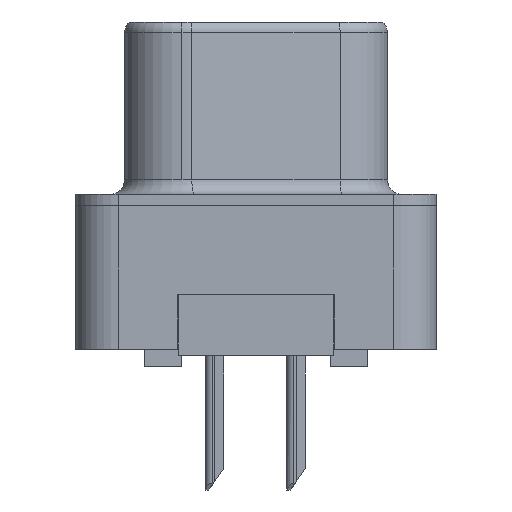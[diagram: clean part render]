
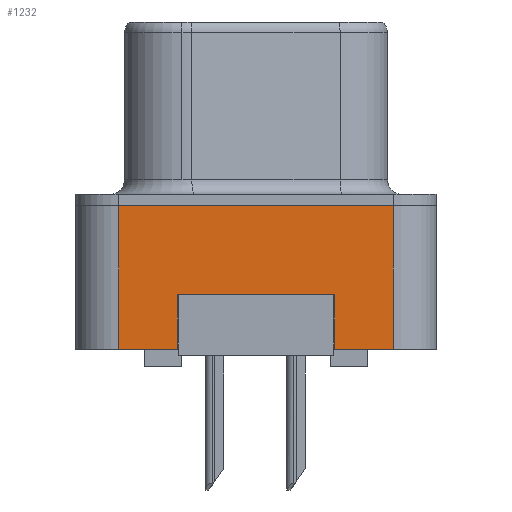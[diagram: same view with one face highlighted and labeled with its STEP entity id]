
A CAD part, left-side view. The second image highlights one B-rep face of the part: STEP entity #1232.
In plain terms, the highlighted planar face has unit normal (-1, 0, 0).
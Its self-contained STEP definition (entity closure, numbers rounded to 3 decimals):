
#212 = CARTESIAN_POINT ( 'NONE',  ( -3., -2.75, -3.1 ) ) ;
#1232 = ADVANCED_FACE ( 'NONE', ( #14462 ), #5292, .T. ) ;
#1903 = DIRECTION ( 'NONE',  ( 0., 0., -1. ) ) ;
#2161 = EDGE_CURVE ( 'NONE', #9326, #15924, #23669, .T. ) ;
#2201 = EDGE_CURVE ( 'NONE', #21811, #5890, #8707, .T. ) ;
#2222 = ORIENTED_EDGE ( 'NONE', *, *, #4855, .F. ) ;
#2808 = ORIENTED_EDGE ( 'NONE', *, *, #2161, .T. ) ;
#3086 = CARTESIAN_POINT ( 'NONE',  ( -3., -4.775, -5. ) ) ;
#3478 = VERTEX_POINT ( 'NONE', #15378 ) ;
#3580 = CARTESIAN_POINT ( 'NONE',  ( -3., 4.775, -5. ) ) ;
#3898 = ORIENTED_EDGE ( 'NONE', *, *, #20613, .T. ) ;
#4206 = DIRECTION ( 'NONE',  ( 0., -1., 0. ) ) ;
#4207 = CARTESIAN_POINT ( 'NONE',  ( -3., 4.775, -5. ) ) ;
#4543 = DIRECTION ( 'NONE',  ( 0., -1., 0. ) ) ;
#4855 = EDGE_CURVE ( 'NONE', #9326, #3478, #13687, .T. ) ;
#5292 = PLANE ( 'NONE',  #23147 ) ;
#5328 = ORIENTED_EDGE ( 'NONE', *, *, #14729, .F. ) ;
#5890 = VERTEX_POINT ( 'NONE', #11511 ) ;
#6472 = VERTEX_POINT ( 'NONE', #3580 ) ;
#7315 = VECTOR ( 'NONE', #11886, 1000. ) ;
#8707 = LINE ( 'NONE', #16070, #13451 ) ;
#8901 = CARTESIAN_POINT ( 'NONE',  ( -3., -4.775, -5. ) ) ;
#9162 = LINE ( 'NONE', #14600, #19308 ) ;
#9326 = VERTEX_POINT ( 'NONE', #212 ) ;
#9876 = LINE ( 'NONE', #15428, #13224 ) ;
#9992 = LINE ( 'NONE', #4207, #16494 ) ;
#11348 = EDGE_LOOP ( 'NONE', ( #2808, #12873, #16657, #22476, #5328, #3898, #13068, #2222 ) ) ;
#11511 = CARTESIAN_POINT ( 'NONE',  ( -3., -4.775, 0. ) ) ;
#11766 = CARTESIAN_POINT ( 'NONE',  ( -3., 2.75, -3.1 ) ) ;
#11886 = DIRECTION ( 'NONE',  ( 0., 1., 0. ) ) ;
#12662 = DIRECTION ( 'NONE',  ( 0., -1., 0. ) ) ;
#12873 = ORIENTED_EDGE ( 'NONE', *, *, #17769, .T. ) ;
#13068 = ORIENTED_EDGE ( 'NONE', *, *, #22928, .F. ) ;
#13224 = VECTOR ( 'NONE', #4206, 1000. ) ;
#13404 = CARTESIAN_POINT ( 'NONE',  ( -3., 4.775, 0. ) ) ;
#13451 = VECTOR ( 'NONE', #23436, 1000. ) ;
#13486 = CARTESIAN_POINT ( 'NONE',  ( -3., -2.75, -5. ) ) ;
#13687 = LINE ( 'NONE', #11766, #7315 ) ;
#14462 = FACE_OUTER_BOUND ( 'NONE', #11348, .T. ) ;
#14600 = CARTESIAN_POINT ( 'NONE',  ( -3., -4.775, -5. ) ) ;
#14729 = EDGE_CURVE ( 'NONE', #6472, #18802, #9992, .T. ) ;
#15378 = CARTESIAN_POINT ( 'NONE',  ( -3., 2.75, -3.1 ) ) ;
#15428 = CARTESIAN_POINT ( 'NONE',  ( -3., -4.775, 0. ) ) ;
#15924 = VERTEX_POINT ( 'NONE', #13486 ) ;
#16037 = DIRECTION ( 'NONE',  ( 0., 0., 1. ) ) ;
#16068 = CARTESIAN_POINT ( 'NONE',  ( -3., 2.75, -3.1 ) ) ;
#16070 = CARTESIAN_POINT ( 'NONE',  ( -3., -4.775, -5. ) ) ;
#16186 = DIRECTION ( 'NONE',  ( 0., 0., -1. ) ) ;
#16373 = VECTOR ( 'NONE', #1903, 1000. ) ;
#16494 = VECTOR ( 'NONE', #16885, 1000. ) ;
#16519 = VERTEX_POINT ( 'NONE', #19493 ) ;
#16657 = ORIENTED_EDGE ( 'NONE', *, *, #2201, .T. ) ;
#16885 = DIRECTION ( 'NONE',  ( 0., 0., 1. ) ) ;
#17769 = EDGE_CURVE ( 'NONE', #15924, #21811, #9162, .T. ) ;
#17886 = LINE ( 'NONE', #16068, #16373 ) ;
#18802 = VERTEX_POINT ( 'NONE', #13404 ) ;
#19002 = VECTOR ( 'NONE', #16186, 1000. ) ;
#19308 = VECTOR ( 'NONE', #12662, 1000. ) ;
#19493 = CARTESIAN_POINT ( 'NONE',  ( -3., 2.75, -5. ) ) ;
#19618 = LINE ( 'NONE', #3086, #22501 ) ;
#19919 = EDGE_CURVE ( 'NONE', #18802, #5890, #9876, .T. ) ;
#20003 = DIRECTION ( 'NONE',  ( -1., 0., 0. ) ) ;
#20613 = EDGE_CURVE ( 'NONE', #6472, #16519, #19618, .T. ) ;
#21731 = CARTESIAN_POINT ( 'NONE',  ( -3., -2.75, -3.1 ) ) ;
#21811 = VERTEX_POINT ( 'NONE', #22760 ) ;
#22476 = ORIENTED_EDGE ( 'NONE', *, *, #19919, .F. ) ;
#22501 = VECTOR ( 'NONE', #4543, 1000. ) ;
#22760 = CARTESIAN_POINT ( 'NONE',  ( -3., -4.775, -5. ) ) ;
#22928 = EDGE_CURVE ( 'NONE', #3478, #16519, #17886, .T. ) ;
#23147 = AXIS2_PLACEMENT_3D ( 'NONE', #8901, #20003, #16037 ) ;
#23436 = DIRECTION ( 'NONE',  ( 0., 0., 1. ) ) ;
#23669 = LINE ( 'NONE', #21731, #19002 ) ;
